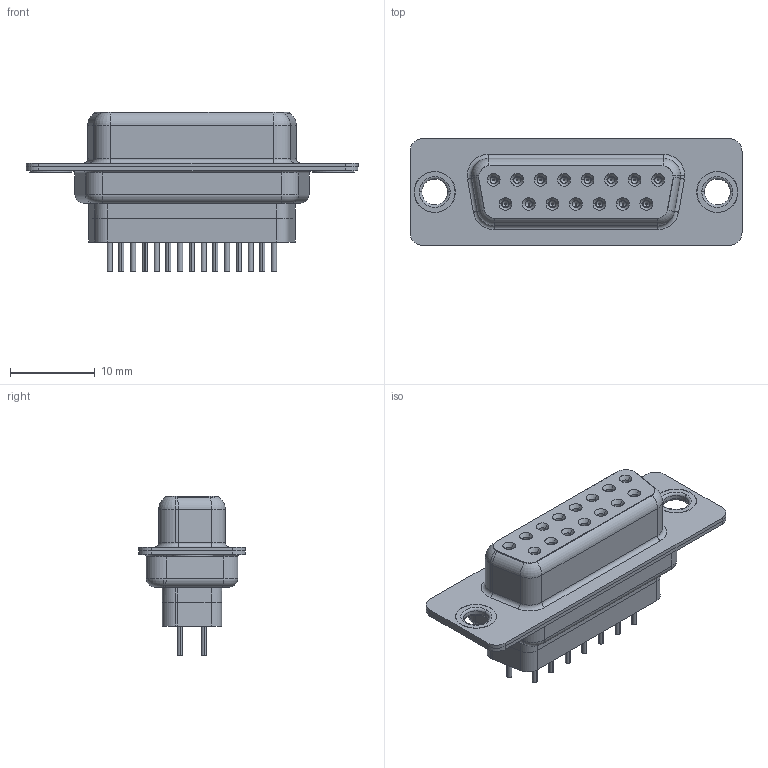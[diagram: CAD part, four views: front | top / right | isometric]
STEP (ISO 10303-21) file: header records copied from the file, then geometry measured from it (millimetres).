
FILE_DESCRIPTION (( 'STEP AP203' ), '1' );
FILE_NAME ('628-015-228-041.STEP', '2020-07-20T22:58:55', ( '' ), ( '' ), 'SwSTEP 2.0', 'SolidWorks 2020', '' );
FILE_SCHEMA (( 'CONFIG_CONTROL_DESIGN' ));
Length unit declared in the file: millimetre
Products named in the file (7): 628 Contact Row 2_28L; 628 Housing_15 FF; 628 Contact Row 1_28L; 628-015-228-041; 628 Shell Front_15 Contacts; 628 Shell Rear_15 Contacts; 628 Thru Hole Rivet
Assembly tree (20 placements, depth 2):
  628-015-228-041
    628 Housing_15 FF
    628 Shell Front_15 Contacts
    628 Shell Rear_15 Contacts
    628 Contact Row 1_28L  x8
    628 Contact Row 2_28L  x7
    628 Thru Hole Rivet  x2
Bounding box: 39.15 x 12.6 x 18.8 mm (x, y, z)
Volume: 2838.8 mm3; surface area: 6891.5 mm2
Topology: 21 solids, 21 shells, 2199 faces, 5580 edges, 3464 vertices
Faces by surface type: cylinder 651, plane 538, torus 455, bspline 300, cone 255
Entity records: 23633 total; most frequent: CARTESIAN_POINT 6002, DIRECTION 3626, ORIENTED_EDGE 3364, EDGE_CURVE 1682, AXIS2_PLACEMENT_3D 1511, VERTEX_POINT 1057, CIRCLE 835, EDGE_LOOP 821
